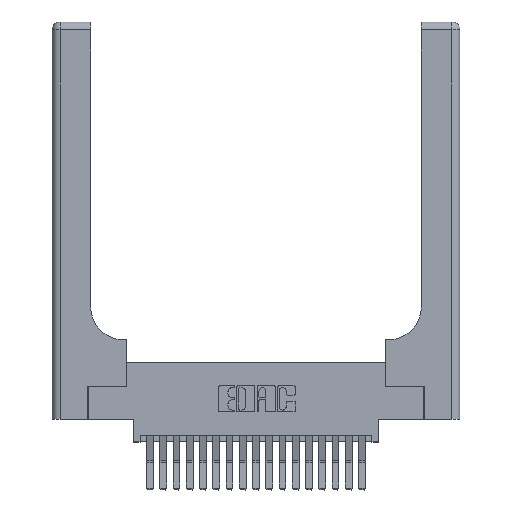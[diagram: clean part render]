
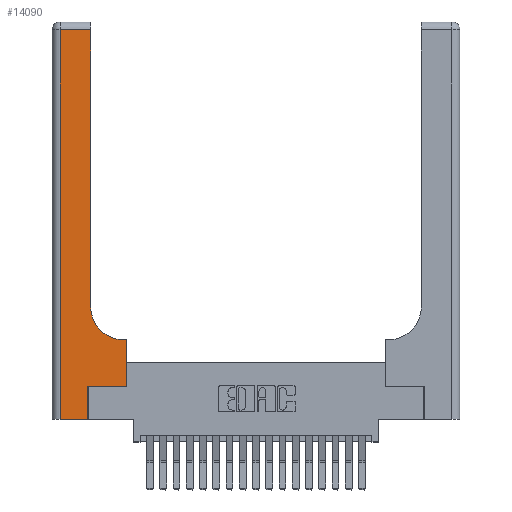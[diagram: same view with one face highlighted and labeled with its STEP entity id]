
A CAD part, top view. The second image highlights one B-rep face of the part: STEP entity #14090.
In plain terms, the highlighted planar face has unit normal (0, 0, 1).
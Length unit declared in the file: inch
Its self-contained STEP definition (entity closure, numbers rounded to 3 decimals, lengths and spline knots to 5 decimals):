
#230 = DIRECTION ( 'NONE',  ( 0., 1., 0. ) ) ;
#376 = CIRCLE ( 'NONE', #6571, 0.25 ) ;
#387 = VECTOR ( 'NONE', #13744, 39.37008 ) ;
#454 = LINE ( 'NONE', #10945, #9135 ) ;
#614 = CARTESIAN_POINT ( 'NONE',  ( 0., 3., 0.37 ) ) ;
#964 = CARTESIAN_POINT ( 'NONE',  ( 0.269, 0.25, 0.37 ) ) ;
#1318 = CARTESIAN_POINT ( 'NONE',  ( 0., 2.94, 0.37 ) ) ;
#1612 = VERTEX_POINT ( 'NONE', #6996 ) ;
#1886 = EDGE_CURVE ( 'NONE', #9649, #19218, #376, .T. ) ;
#1959 = CARTESIAN_POINT ( 'NONE',  ( 0.5415, 0.6, 0.37 ) ) ;
#2001 = ORIENTED_EDGE ( 'NONE', *, *, #16960, .T. ) ;
#2092 = FACE_OUTER_BOUND ( 'NONE', #9392, .T. ) ;
#2251 = EDGE_CURVE ( 'NONE', #14212, #16877, #3788, .T. ) ;
#2825 = ORIENTED_EDGE ( 'NONE', *, *, #3653, .T. ) ;
#3010 = CARTESIAN_POINT ( 'NONE',  ( 0.2915, 0.6, 0.37 ) ) ;
#3057 = DIRECTION ( 'NONE',  ( -1., 0., 0. ) ) ;
#3228 = VECTOR ( 'NONE', #230, 39.37008 ) ;
#3477 = ORIENTED_EDGE ( 'NONE', *, *, #2251, .T. ) ;
#3569 = CARTESIAN_POINT ( 'NONE',  ( 0., 0., 0.37 ) ) ;
#3653 = EDGE_CURVE ( 'NONE', #16877, #4779, #3725, .T. ) ;
#3725 = LINE ( 'NONE', #5999, #8331 ) ;
#3788 = LINE ( 'NONE', #8881, #3228 ) ;
#4147 = DIRECTION ( 'NONE',  ( -1., 0., 0. ) ) ;
#4529 = DIRECTION ( 'NONE',  ( 0., 0., -1. ) ) ;
#4779 = VERTEX_POINT ( 'NONE', #7391 ) ;
#5087 = CARTESIAN_POINT ( 'NONE',  ( 0.5585, 0.6, 0.37 ) ) ;
#5551 = CARTESIAN_POINT ( 'NONE',  ( 0.2915, 2.94, 0.37 ) ) ;
#5632 = EDGE_CURVE ( 'NONE', #4779, #14425, #20639, .T. ) ;
#5999 = CARTESIAN_POINT ( 'NONE',  ( 0.269, 0.25, 0.37 ) ) ;
#6571 = AXIS2_PLACEMENT_3D ( 'NONE', #14733, #4529, #16425 ) ;
#6996 = CARTESIAN_POINT ( 'NONE',  ( 0.06, 0., 0.37 ) ) ;
#7183 = VECTOR ( 'NONE', #14660, 39.37008 ) ;
#7391 = CARTESIAN_POINT ( 'NONE',  ( 0.5585, 0.25, 0.37 ) ) ;
#7423 = ORIENTED_EDGE ( 'NONE', *, *, #5632, .T. ) ;
#8331 = VECTOR ( 'NONE', #19487, 39.37008 ) ;
#8336 = CARTESIAN_POINT ( 'NONE',  ( 0.06, 2.94, 0.37 ) ) ;
#8409 = VERTEX_POINT ( 'NONE', #5551 ) ;
#8538 = VECTOR ( 'NONE', #20599, 39.37008 ) ;
#8815 = CARTESIAN_POINT ( 'NONE',  ( 0.2915, 3., 0.37 ) ) ;
#8881 = CARTESIAN_POINT ( 'NONE',  ( 0.269, 0., 0.37 ) ) ;
#8953 = EDGE_CURVE ( 'NONE', #19218, #8409, #12522, .T. ) ;
#9135 = VECTOR ( 'NONE', #19310, 39.37008 ) ;
#9392 = EDGE_LOOP ( 'NONE', ( #16095, #11237, #16577, #11751, #3477, #2825, #7423, #2001, #14095 ) ) ;
#9628 = CARTESIAN_POINT ( 'NONE',  ( 0.269, 0., 0.37 ) ) ;
#9649 = VERTEX_POINT ( 'NONE', #1959 ) ;
#10704 = VECTOR ( 'NONE', #3057, 39.37008 ) ;
#10945 = CARTESIAN_POINT ( 'NONE',  ( 0.06, 3., 0.37 ) ) ;
#11237 = ORIENTED_EDGE ( 'NONE', *, *, #20895, .T. ) ;
#11386 = LINE ( 'NONE', #3010, #20853 ) ;
#11751 = ORIENTED_EDGE ( 'NONE', *, *, #21480, .T. ) ;
#12254 = CARTESIAN_POINT ( 'NONE',  ( 0.2915, 0.85, 0.37 ) ) ;
#12522 = LINE ( 'NONE', #8815, #8538 ) ;
#12978 = CARTESIAN_POINT ( 'NONE',  ( 0.5585, 0.25, 0.37 ) ) ;
#13744 = DIRECTION ( 'NONE',  ( 1., 0., 0. ) ) ;
#14090 = ADVANCED_FACE ( 'NONE', ( #2092 ), #21055, .F. ) ;
#14095 = ORIENTED_EDGE ( 'NONE', *, *, #1886, .T. ) ;
#14212 = VERTEX_POINT ( 'NONE', #9628 ) ;
#14358 = DIRECTION ( 'NONE',  ( 0., 0., -1. ) ) ;
#14425 = VERTEX_POINT ( 'NONE', #5087 ) ;
#14660 = DIRECTION ( 'NONE',  ( 0., 1., 0. ) ) ;
#14733 = CARTESIAN_POINT ( 'NONE',  ( 0.5415, 0.85, 0.37 ) ) ;
#14999 = DIRECTION ( 'NONE',  ( -1., 0., 0. ) ) ;
#16095 = ORIENTED_EDGE ( 'NONE', *, *, #8953, .T. ) ;
#16425 = DIRECTION ( 'NONE',  ( 1., 0., 0. ) ) ;
#16577 = ORIENTED_EDGE ( 'NONE', *, *, #19984, .T. ) ;
#16877 = VERTEX_POINT ( 'NONE', #964 ) ;
#16960 = EDGE_CURVE ( 'NONE', #14425, #9649, #11386, .T. ) ;
#17519 = LINE ( 'NONE', #3569, #387 ) ;
#19218 = VERTEX_POINT ( 'NONE', #12254 ) ;
#19310 = DIRECTION ( 'NONE',  ( 0., -1., 0. ) ) ;
#19487 = DIRECTION ( 'NONE',  ( 1., 0., 0. ) ) ;
#19639 = LINE ( 'NONE', #1318, #10704 ) ;
#19984 = EDGE_CURVE ( 'NONE', #20328, #1612, #454, .T. ) ;
#20328 = VERTEX_POINT ( 'NONE', #8336 ) ;
#20599 = DIRECTION ( 'NONE',  ( 0., 1., 0. ) ) ;
#20639 = LINE ( 'NONE', #12978, #7183 ) ;
#20853 = VECTOR ( 'NONE', #14999, 39.37008 ) ;
#20895 = EDGE_CURVE ( 'NONE', #8409, #20328, #19639, .T. ) ;
#21055 = PLANE ( 'NONE',  #21251 ) ;
#21251 = AXIS2_PLACEMENT_3D ( 'NONE', #614, #14358, #4147 ) ;
#21480 = EDGE_CURVE ( 'NONE', #1612, #14212, #17519, .T. ) ;
